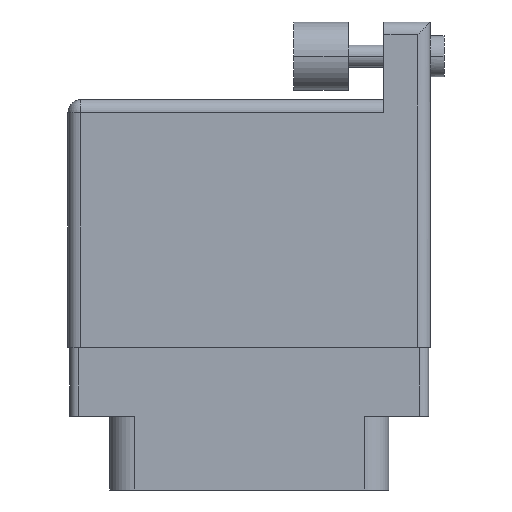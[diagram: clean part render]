
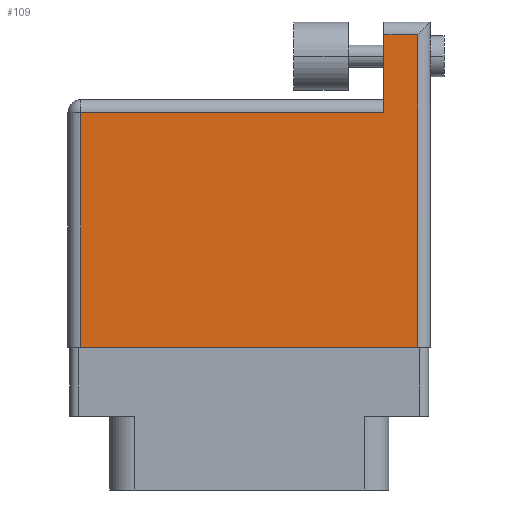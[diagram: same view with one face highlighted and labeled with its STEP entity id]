
A CAD part, front view. The second image highlights one B-rep face of the part: STEP entity #109.
In plain terms, the highlighted face is planar.
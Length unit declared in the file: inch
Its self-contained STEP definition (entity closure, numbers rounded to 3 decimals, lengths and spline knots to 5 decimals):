
#109 = ADVANCED_FACE ( 'NONE', ( #16765 ), #7535, .F. ) ;
#463 = CARTESIAN_POINT ( 'NONE',  ( 1.278, 1.143, 0. ) ) ;
#982 = ORIENTED_EDGE ( 'NONE', *, *, #7285, .T. ) ;
#1235 = ORIENTED_EDGE ( 'NONE', *, *, #7175, .T. ) ;
#1338 = CARTESIAN_POINT ( 'NONE',  ( 1.155, 1.19, 0. ) ) ;
#2223 = ORIENTED_EDGE ( 'NONE', *, *, #5502, .T. ) ;
#2448 = VECTOR ( 'NONE', #12516, 39.37008 ) ;
#2880 = LINE ( 'NONE', #18254, #2448 ) ;
#3289 = DIRECTION ( 'NONE',  ( 0., -1., 0. ) ) ;
#3754 = CARTESIAN_POINT ( 'NONE',  ( 1.278, 0., 0. ) ) ;
#4293 = VECTOR ( 'NONE', #10819, 39.37008 ) ;
#4349 = ORIENTED_EDGE ( 'NONE', *, *, #12763, .T. ) ;
#4701 = EDGE_CURVE ( 'NONE', #10128, #14284, #16141, .T. ) ;
#4754 = ORIENTED_EDGE ( 'NONE', *, *, #7851, .T. ) ;
#5211 = LINE ( 'NONE', #13978, #4293 ) ;
#5447 = VERTEX_POINT ( 'NONE', #17800 ) ;
#5502 = EDGE_CURVE ( 'NONE', #11231, #5447, #10924, .T. ) ;
#5630 = DIRECTION ( 'NONE',  ( -1., 0., 0. ) ) ;
#6164 = CARTESIAN_POINT ( 'NONE',  ( 1.155, 0.859, 0. ) ) ;
#7163 = EDGE_LOOP ( 'NONE', ( #4349, #1235, #14026, #4754, #982, #2223 ) ) ;
#7175 = EDGE_CURVE ( 'NONE', #17283, #10128, #9474, .T. ) ;
#7285 = EDGE_CURVE ( 'NONE', #18271, #11231, #2880, .T. ) ;
#7426 = VECTOR ( 'NONE', #3289, 39.37008 ) ;
#7504 = CARTESIAN_POINT ( 'NONE',  ( 1.278, 1.19, 0. ) ) ;
#7535 = PLANE ( 'NONE',  #17861 ) ;
#7851 = EDGE_CURVE ( 'NONE', #14284, #18271, #11311, .T. ) ;
#8570 = VECTOR ( 'NONE', #10625, 39.37008 ) ;
#8810 = DIRECTION ( 'NONE',  ( -1., 0., 0. ) ) ;
#9040 = CARTESIAN_POINT ( 'NONE',  ( 0.047, 0., 0. ) ) ;
#9104 = CARTESIAN_POINT ( 'NONE',  ( 1.155, 1.143, 0. ) ) ;
#9474 = LINE ( 'NONE', #7504, #8570 ) ;
#9898 = CARTESIAN_POINT ( 'NONE',  ( 1.155, 1.143, 0. ) ) ;
#10128 = VERTEX_POINT ( 'NONE', #463 ) ;
#10342 = CARTESIAN_POINT ( 'NONE',  ( 0., 0.906, 0. ) ) ;
#10625 = DIRECTION ( 'NONE',  ( 0., 1., 0. ) ) ;
#10819 = DIRECTION ( 'NONE',  ( 1., 0., 0. ) ) ;
#10924 = LINE ( 'NONE', #9040, #18642 ) ;
#11231 = VERTEX_POINT ( 'NONE', #13039 ) ;
#11311 = LINE ( 'NONE', #1338, #7426 ) ;
#12278 = VECTOR ( 'NONE', #5630, 39.37008 ) ;
#12516 = DIRECTION ( 'NONE',  ( -1., 0., 0. ) ) ;
#12763 = EDGE_CURVE ( 'NONE', #5447, #17283, #5211, .T. ) ;
#13039 = CARTESIAN_POINT ( 'NONE',  ( 0.047, 0.859, 0. ) ) ;
#13978 = CARTESIAN_POINT ( 'NONE',  ( 0., 0., 0. ) ) ;
#14026 = ORIENTED_EDGE ( 'NONE', *, *, #4701, .T. ) ;
#14284 = VERTEX_POINT ( 'NONE', #9104 ) ;
#14781 = DIRECTION ( 'NONE',  ( 0., 0., -1. ) ) ;
#16141 = LINE ( 'NONE', #9898, #12278 ) ;
#16323 = DIRECTION ( 'NONE',  ( 0., -1., 0. ) ) ;
#16765 = FACE_OUTER_BOUND ( 'NONE', #7163, .T. ) ;
#17283 = VERTEX_POINT ( 'NONE', #3754 ) ;
#17800 = CARTESIAN_POINT ( 'NONE',  ( 0.047, 0., 0. ) ) ;
#17861 = AXIS2_PLACEMENT_3D ( 'NONE', #10342, #14781, #8810 ) ;
#18254 = CARTESIAN_POINT ( 'NONE',  ( 0., 0.859, 0. ) ) ;
#18271 = VERTEX_POINT ( 'NONE', #6164 ) ;
#18642 = VECTOR ( 'NONE', #16323, 39.37008 ) ;
